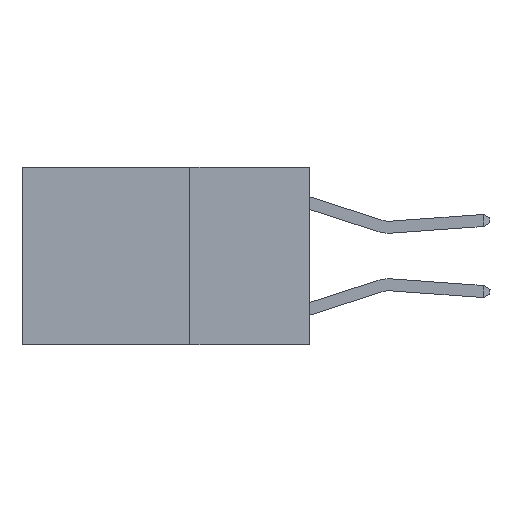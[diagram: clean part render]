
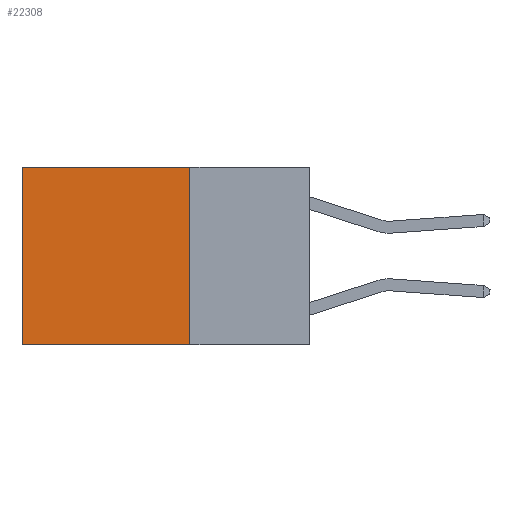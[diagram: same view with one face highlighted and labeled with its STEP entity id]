
A CAD part, left-side view. The second image highlights one B-rep face of the part: STEP entity #22308.
In plain terms, the highlighted planar face has unit normal (-1, 0, 0).
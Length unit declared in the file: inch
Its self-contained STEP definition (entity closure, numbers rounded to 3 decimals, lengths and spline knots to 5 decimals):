
#168 = VECTOR ( 'NONE', #14693, 39.37008 ) ;
#368 = EDGE_CURVE ( 'NONE', #16385, #9783, #22886, .T. ) ;
#638 = VECTOR ( 'NONE', #16584, 39.37008 ) ;
#837 = LINE ( 'NONE', #2126, #168 ) ;
#2126 = CARTESIAN_POINT ( 'NONE',  ( 0.2625, 0.25, -0.37 ) ) ;
#2373 = CARTESIAN_POINT ( 'NONE',  ( 0.2625, 0.6, 0. ) ) ;
#3297 = ORIENTED_EDGE ( 'NONE', *, *, #3412, .F. ) ;
#3340 = VERTEX_POINT ( 'NONE', #18701 ) ;
#3412 = EDGE_CURVE ( 'NONE', #3340, #9783, #837, .T. ) ;
#3763 = CARTESIAN_POINT ( 'NONE',  ( 0.2625, 0.25, 0. ) ) ;
#4270 = CARTESIAN_POINT ( 'NONE',  ( 0.2625, 0.6, -0.37 ) ) ;
#6572 = DIRECTION ( 'NONE',  ( 0., 1., 0. ) ) ;
#8889 = EDGE_LOOP ( 'NONE', ( #24825, #3297, #26452, #12671 ) ) ;
#9783 = VERTEX_POINT ( 'NONE', #4270 ) ;
#10150 = DIRECTION ( 'NONE',  ( 1., 0., 0. ) ) ;
#10796 = CARTESIAN_POINT ( 'NONE',  ( 0.2625, 0.25, 0. ) ) ;
#11059 = LINE ( 'NONE', #26099, #22090 ) ;
#11265 = VERTEX_POINT ( 'NONE', #13047 ) ;
#11544 = DIRECTION ( 'NONE',  ( 0., 0., -1. ) ) ;
#12269 = FACE_OUTER_BOUND ( 'NONE', #8889, .T. ) ;
#12671 = ORIENTED_EDGE ( 'NONE', *, *, #15603, .T. ) ;
#13047 = CARTESIAN_POINT ( 'NONE',  ( 0.2625, 0.25, 0. ) ) ;
#14693 = DIRECTION ( 'NONE',  ( 0., 1., 0. ) ) ;
#15603 = EDGE_CURVE ( 'NONE', #11265, #16385, #19560, .T. ) ;
#16385 = VERTEX_POINT ( 'NONE', #2373 ) ;
#16584 = DIRECTION ( 'NONE',  ( 0., 0., -1. ) ) ;
#18701 = CARTESIAN_POINT ( 'NONE',  ( 0.2625, 0.25, -0.37 ) ) ;
#19560 = LINE ( 'NONE', #10796, #20843 ) ;
#20480 = EDGE_CURVE ( 'NONE', #11265, #3340, #11059, .T. ) ;
#20843 = VECTOR ( 'NONE', #6572, 39.37008 ) ;
#22090 = VECTOR ( 'NONE', #11544, 39.37008 ) ;
#22308 = ADVANCED_FACE ( 'NONE', ( #12269 ), #22554, .F. ) ;
#22554 = PLANE ( 'NONE',  #23249 ) ;
#22741 = CARTESIAN_POINT ( 'NONE',  ( 0.2625, 0.6, 0. ) ) ;
#22886 = LINE ( 'NONE', #22741, #638 ) ;
#23249 = AXIS2_PLACEMENT_3D ( 'NONE', #3763, #10150, #24611 ) ;
#24611 = DIRECTION ( 'NONE',  ( 0., 0., -1. ) ) ;
#24825 = ORIENTED_EDGE ( 'NONE', *, *, #368, .T. ) ;
#26099 = CARTESIAN_POINT ( 'NONE',  ( 0.2625, 0.25, 0. ) ) ;
#26452 = ORIENTED_EDGE ( 'NONE', *, *, #20480, .F. ) ;
